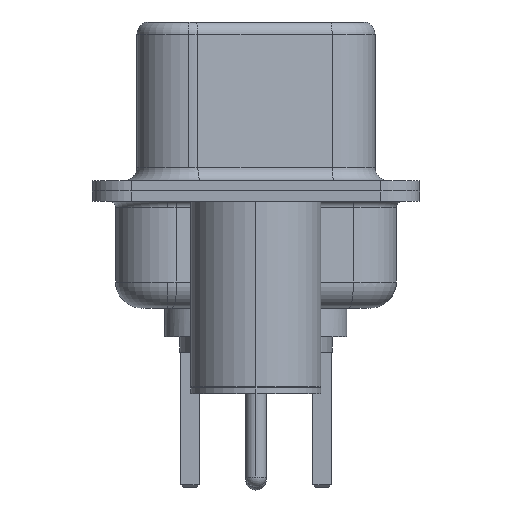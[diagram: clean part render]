
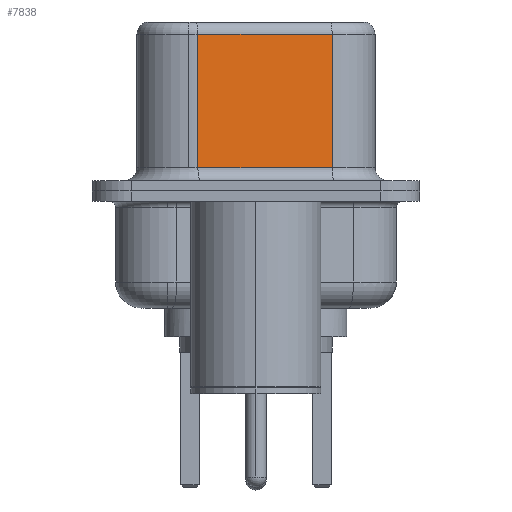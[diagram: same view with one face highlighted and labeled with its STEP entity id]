
A CAD part, left-side view. The second image highlights one B-rep face of the part: STEP entity #7838.
In plain terms, the highlighted planar face has unit normal (-0.985, -0.174, 0).
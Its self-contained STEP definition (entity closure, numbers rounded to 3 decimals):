
#181 = DIRECTION ( 'NONE',  ( 0., 0., -1. ) ) ;
#1437 = VECTOR ( 'NONE', #181, 1000. ) ;
#2236 = CARTESIAN_POINT ( 'NONE',  ( 3.655, 2.233, 6.52 ) ) ;
#2685 = EDGE_CURVE ( 'NONE', #10101, #18346, #17285, .T. ) ;
#2843 = PLANE ( 'NONE',  #6379 ) ;
#3833 = EDGE_CURVE ( 'NONE', #17579, #15176, #8529, .T. ) ;
#4036 = EDGE_CURVE ( 'NONE', #17579, #18346, #9703, .T. ) ;
#4323 = VECTOR ( 'NONE', #17414, 1000. ) ;
#4871 = CARTESIAN_POINT ( 'NONE',  ( 4.565, -2.927, 0.9 ) ) ;
#4949 = ORIENTED_EDGE ( 'NONE', *, *, #2685, .T. ) ;
#5882 = CARTESIAN_POINT ( 'NONE',  ( 4.565, -2.927, 6.52 ) ) ;
#6379 = AXIS2_PLACEMENT_3D ( 'NONE', #5882, #18342, #9058 ) ;
#6867 = DIRECTION ( 'NONE',  ( 0., 0., -1. ) ) ;
#7397 = ORIENTED_EDGE ( 'NONE', *, *, #4036, .F. ) ;
#7838 = ADVANCED_FACE ( 'NONE', ( #16752 ), #2843, .F. ) ;
#7994 = LINE ( 'NONE', #2236, #15756 ) ;
#8529 = LINE ( 'NONE', #8570, #4323 ) ;
#8570 = CARTESIAN_POINT ( 'NONE',  ( 4.565, -2.927, 6.02 ) ) ;
#8908 = DIRECTION ( 'NONE',  ( 0.174, -0.985, 0. ) ) ;
#9058 = DIRECTION ( 'NONE',  ( -0.174, 0.985, 0. ) ) ;
#9613 = CARTESIAN_POINT ( 'NONE',  ( 4.565, -2.927, 6.52 ) ) ;
#9703 = LINE ( 'NONE', #9613, #1437 ) ;
#10101 = VERTEX_POINT ( 'NONE', #14465 ) ;
#12428 = ORIENTED_EDGE ( 'NONE', *, *, #16599, .T. ) ;
#12626 = VECTOR ( 'NONE', #8908, 1000. ) ;
#13766 = CARTESIAN_POINT ( 'NONE',  ( 4.565, -2.927, 6.02 ) ) ;
#13861 = EDGE_LOOP ( 'NONE', ( #7397, #16158, #12428, #4949 ) ) ;
#14465 = CARTESIAN_POINT ( 'NONE',  ( 3.655, 2.233, 0.9 ) ) ;
#15176 = VERTEX_POINT ( 'NONE', #15806 ) ;
#15756 = VECTOR ( 'NONE', #6867, 1000. ) ;
#15801 = CARTESIAN_POINT ( 'NONE',  ( 4.565, -2.927, 0.9 ) ) ;
#15806 = CARTESIAN_POINT ( 'NONE',  ( 3.655, 2.233, 6.02 ) ) ;
#16158 = ORIENTED_EDGE ( 'NONE', *, *, #3833, .T. ) ;
#16599 = EDGE_CURVE ( 'NONE', #15176, #10101, #7994, .T. ) ;
#16752 = FACE_OUTER_BOUND ( 'NONE', #13861, .T. ) ;
#17285 = LINE ( 'NONE', #15801, #12626 ) ;
#17414 = DIRECTION ( 'NONE',  ( -0.174, 0.985, 0. ) ) ;
#17579 = VERTEX_POINT ( 'NONE', #13766 ) ;
#18342 = DIRECTION ( 'NONE',  ( 0.985, 0.174, 0. ) ) ;
#18346 = VERTEX_POINT ( 'NONE', #4871 ) ;
